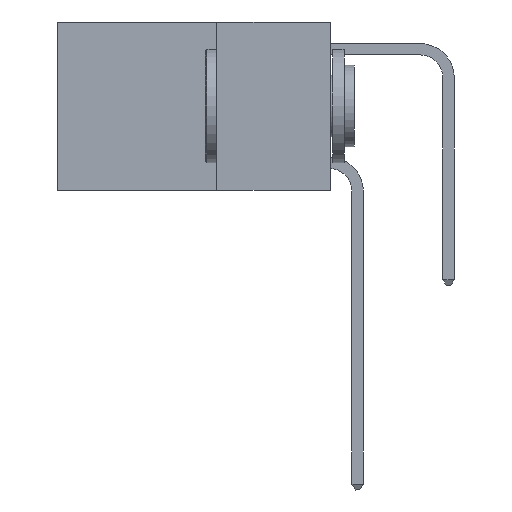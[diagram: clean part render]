
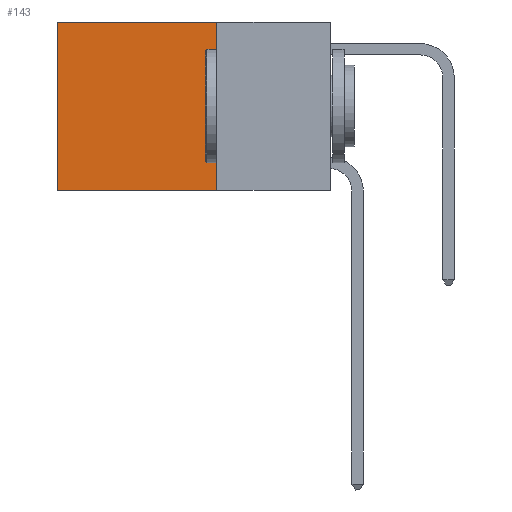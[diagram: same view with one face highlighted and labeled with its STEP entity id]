
A CAD part, left-side view. The second image highlights one B-rep face of the part: STEP entity #143.
In plain terms, the highlighted planar face has unit normal (-1, 0, 0).
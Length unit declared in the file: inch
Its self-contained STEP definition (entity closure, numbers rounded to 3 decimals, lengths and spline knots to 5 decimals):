
#10 = ORIENTED_EDGE ( 'NONE', *, *, #11298, .F. ) ;
#143 = ADVANCED_FACE ( 'NONE', ( #3792 ), #1854, .F. ) ;
#183 = LINE ( 'NONE', #6197, #12142 ) ;
#1129 = DIRECTION ( 'NONE',  ( 0., 0., -1. ) ) ;
#1498 = EDGE_LOOP ( 'NONE', ( #11920, #10, #9058, #12510 ) ) ;
#1854 = PLANE ( 'NONE',  #11267 ) ;
#2067 = DIRECTION ( 'NONE',  ( 0., 1., 0. ) ) ;
#2284 = VERTEX_POINT ( 'NONE', #11669 ) ;
#2755 = VERTEX_POINT ( 'NONE', #11279 ) ;
#2932 = DIRECTION ( 'NONE',  ( 0., 0., -1. ) ) ;
#2990 = LINE ( 'NONE', #11193, #3156 ) ;
#3156 = VECTOR ( 'NONE', #7975, 39.37008 ) ;
#3792 = FACE_OUTER_BOUND ( 'NONE', #1498, .T. ) ;
#3868 = DIRECTION ( 'NONE',  ( 1., 0., 0. ) ) ;
#5775 = VECTOR ( 'NONE', #2067, 39.37008 ) ;
#6064 = CARTESIAN_POINT ( 'NONE',  ( 0.2625, 0.25, 0. ) ) ;
#6197 = CARTESIAN_POINT ( 'NONE',  ( 0.2625, 0.6, 0. ) ) ;
#6602 = CARTESIAN_POINT ( 'NONE',  ( 0.2625, 0.6, 0. ) ) ;
#7282 = EDGE_CURVE ( 'NONE', #2284, #12682, #7888, .T. ) ;
#7888 = LINE ( 'NONE', #6064, #11913 ) ;
#7909 = CARTESIAN_POINT ( 'NONE',  ( 0.2625, 0.25, 0. ) ) ;
#7975 = DIRECTION ( 'NONE',  ( 0., 0., -1. ) ) ;
#8062 = EDGE_CURVE ( 'NONE', #2284, #2755, #2990, .T. ) ;
#9058 = ORIENTED_EDGE ( 'NONE', *, *, #8062, .F. ) ;
#10968 = VERTEX_POINT ( 'NONE', #12824 ) ;
#11193 = CARTESIAN_POINT ( 'NONE',  ( 0.2625, 0.25, 0. ) ) ;
#11267 = AXIS2_PLACEMENT_3D ( 'NONE', #7909, #3868, #2932 ) ;
#11279 = CARTESIAN_POINT ( 'NONE',  ( 0.2625, 0.25, -0.37 ) ) ;
#11298 = EDGE_CURVE ( 'NONE', #2755, #10968, #11328, .T. ) ;
#11328 = LINE ( 'NONE', #11459, #5775 ) ;
#11459 = CARTESIAN_POINT ( 'NONE',  ( 0.2625, 0.25, -0.37 ) ) ;
#11669 = CARTESIAN_POINT ( 'NONE',  ( 0.2625, 0.25, 0. ) ) ;
#11913 = VECTOR ( 'NONE', #11958, 39.37008 ) ;
#11920 = ORIENTED_EDGE ( 'NONE', *, *, #12946, .T. ) ;
#11958 = DIRECTION ( 'NONE',  ( 0., 1., 0. ) ) ;
#12142 = VECTOR ( 'NONE', #1129, 39.37008 ) ;
#12510 = ORIENTED_EDGE ( 'NONE', *, *, #7282, .T. ) ;
#12682 = VERTEX_POINT ( 'NONE', #6602 ) ;
#12824 = CARTESIAN_POINT ( 'NONE',  ( 0.2625, 0.6, -0.37 ) ) ;
#12946 = EDGE_CURVE ( 'NONE', #12682, #10968, #183, .T. ) ;
